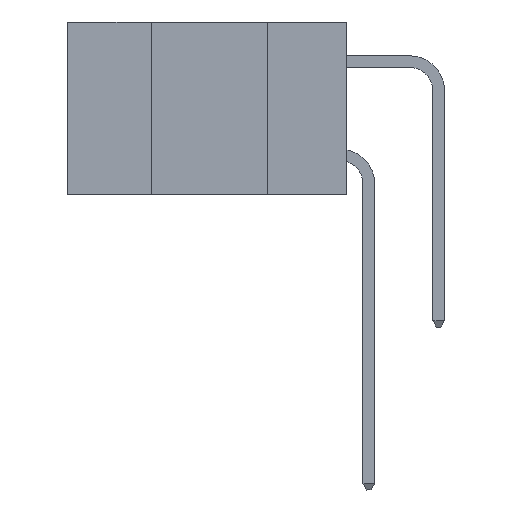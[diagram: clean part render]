
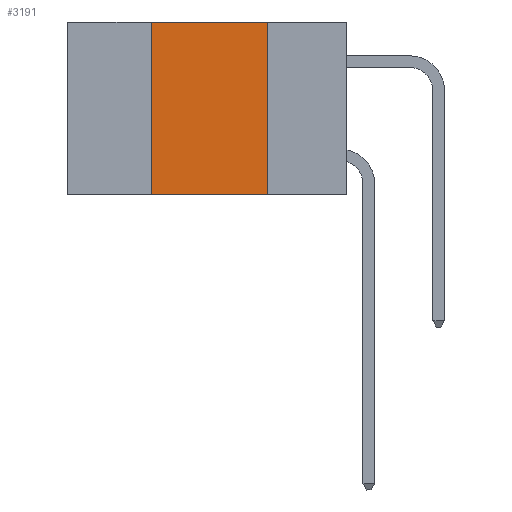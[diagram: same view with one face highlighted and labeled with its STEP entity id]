
A CAD part, left-side view. The second image highlights one B-rep face of the part: STEP entity #3191.
In plain terms, the highlighted planar face has unit normal (-1, 0, 0).
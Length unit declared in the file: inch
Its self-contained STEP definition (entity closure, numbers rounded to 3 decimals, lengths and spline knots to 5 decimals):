
#525 = ORIENTED_EDGE ( 'NONE', *, *, #14987, .F. ) ;
#2211 = VERTEX_POINT ( 'NONE', #5929 ) ;
#2574 = EDGE_CURVE ( 'NONE', #17185, #2211, #9585, .T. ) ;
#3191 = ADVANCED_FACE ( 'NONE', ( #10867 ), #11154, .F. ) ;
#4016 = LINE ( 'NONE', #12838, #20695 ) ;
#4588 = CARTESIAN_POINT ( 'NONE',  ( 0., 0.6, 0. ) ) ;
#4641 = DIRECTION ( 'NONE',  ( 0., -1., 0. ) ) ;
#5929 = CARTESIAN_POINT ( 'NONE',  ( 0., 0.17, -0.37 ) ) ;
#6050 = VERTEX_POINT ( 'NONE', #19950 ) ;
#6184 = DIRECTION ( 'NONE',  ( 0., 0., -1. ) ) ;
#6266 = DIRECTION ( 'NONE',  ( 1., 0., 0. ) ) ;
#6321 = CARTESIAN_POINT ( 'NONE',  ( 0., 0.6, 0. ) ) ;
#7226 = LINE ( 'NONE', #6321, #15670 ) ;
#7791 = CARTESIAN_POINT ( 'NONE',  ( 0., 0.42, 0. ) ) ;
#9585 = LINE ( 'NONE', #19494, #17998 ) ;
#9948 = LINE ( 'NONE', #17252, #18350 ) ;
#10431 = EDGE_CURVE ( 'NONE', #17185, #14439, #9948, .T. ) ;
#10867 = FACE_OUTER_BOUND ( 'NONE', #11958, .T. ) ;
#10886 = ORIENTED_EDGE ( 'NONE', *, *, #17643, .F. ) ;
#11154 = PLANE ( 'NONE',  #21647 ) ;
#11958 = EDGE_LOOP ( 'NONE', ( #525, #10886, #18498, #15950 ) ) ;
#12838 = CARTESIAN_POINT ( 'NONE',  ( 0., 0.17, 0. ) ) ;
#14439 = VERTEX_POINT ( 'NONE', #7791 ) ;
#14987 = EDGE_CURVE ( 'NONE', #6050, #2211, #4016, .T. ) ;
#15670 = VECTOR ( 'NONE', #4641, 39.37008 ) ;
#15950 = ORIENTED_EDGE ( 'NONE', *, *, #2574, .T. ) ;
#16290 = DIRECTION ( 'NONE',  ( 0., -1., 0. ) ) ;
#17185 = VERTEX_POINT ( 'NONE', #20006 ) ;
#17252 = CARTESIAN_POINT ( 'NONE',  ( 0., 0.42, 0. ) ) ;
#17643 = EDGE_CURVE ( 'NONE', #14439, #6050, #7226, .T. ) ;
#17986 = DIRECTION ( 'NONE',  ( 0., 0., -1. ) ) ;
#17998 = VECTOR ( 'NONE', #16290, 39.37008 ) ;
#18350 = VECTOR ( 'NONE', #18904, 39.37008 ) ;
#18498 = ORIENTED_EDGE ( 'NONE', *, *, #10431, .F. ) ;
#18904 = DIRECTION ( 'NONE',  ( 0., 0., 1. ) ) ;
#19494 = CARTESIAN_POINT ( 'NONE',  ( 0., 0.6, -0.37 ) ) ;
#19950 = CARTESIAN_POINT ( 'NONE',  ( 0., 0.17, 0. ) ) ;
#20006 = CARTESIAN_POINT ( 'NONE',  ( 0., 0.42, -0.37 ) ) ;
#20695 = VECTOR ( 'NONE', #6184, 39.37008 ) ;
#21647 = AXIS2_PLACEMENT_3D ( 'NONE', #4588, #6266, #17986 ) ;
